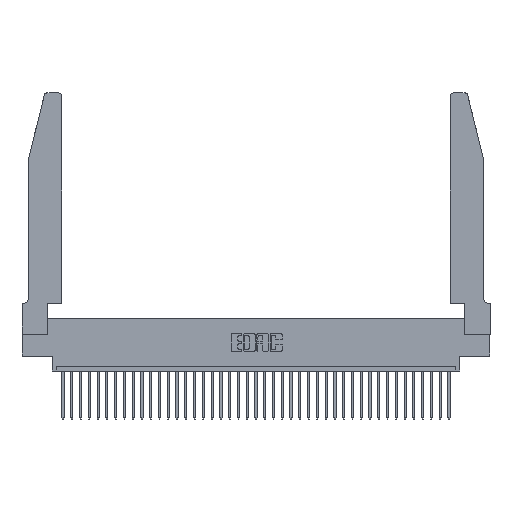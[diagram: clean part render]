
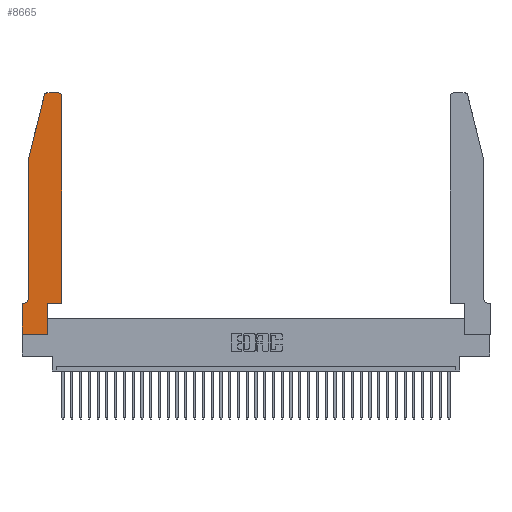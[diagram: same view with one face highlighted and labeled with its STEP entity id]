
A CAD part, top view. The second image highlights one B-rep face of the part: STEP entity #8665.
In plain terms, the highlighted planar face has unit normal (0, 0, 1).
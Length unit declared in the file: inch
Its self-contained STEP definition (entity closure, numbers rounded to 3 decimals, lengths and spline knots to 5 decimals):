
#270 = VECTOR ( 'NONE', #23869, 39.37008 ) ;
#405 = EDGE_LOOP ( 'NONE', ( #17912, #5666, #31619, #15824, #33935, #34351, #32265, #9111, #30380, #34978, #33684, #30118 ) ) ;
#800 = DIRECTION ( 'NONE',  ( -1., 0., 0. ) ) ;
#1045 = FACE_OUTER_BOUND ( 'NONE', #405, .T. ) ;
#1576 = DIRECTION ( 'NONE',  ( 0., 0., 1. ) ) ;
#2291 = DIRECTION ( 'NONE',  ( 1., 0., 0. ) ) ;
#2336 = CARTESIAN_POINT ( 'NONE',  ( 0.0755, 2., 0.37 ) ) ;
#2370 = VERTEX_POINT ( 'NONE', #35701 ) ;
#3829 = EDGE_CURVE ( 'NONE', #26763, #27027, #23783, .T. ) ;
#4012 = DIRECTION ( 'NONE',  ( -1., 0., 0. ) ) ;
#5098 = DIRECTION ( 'NONE',  ( 1., 0., 0. ) ) ;
#5636 = AXIS2_PLACEMENT_3D ( 'NONE', #30112, #15442, #800 ) ;
#5666 = ORIENTED_EDGE ( 'NONE', *, *, #27559, .T. ) ;
#6592 = DIRECTION ( 'NONE',  ( 1., 0., 0. ) ) ;
#6665 = VECTOR ( 'NONE', #4012, 39.37008 ) ;
#6787 = VERTEX_POINT ( 'NONE', #27611 ) ;
#7385 = EDGE_CURVE ( 'NONE', #20689, #2370, #35392, .T. ) ;
#7704 = CARTESIAN_POINT ( 'NONE',  ( 0., 0.35, 0.37 ) ) ;
#7890 = DIRECTION ( 'NONE',  ( 1., 0., 0. ) ) ;
#8224 = LINE ( 'NONE', #18073, #270 ) ;
#8253 = DIRECTION ( 'NONE',  ( 0., 0., 1. ) ) ;
#8665 = ADVANCED_FACE ( 'NONE', ( #1045 ), #26020, .T. ) ;
#9111 = ORIENTED_EDGE ( 'NONE', *, *, #23166, .T. ) ;
#9281 = AXIS2_PLACEMENT_3D ( 'NONE', #11340, #14452, #2291 ) ;
#10300 = CIRCLE ( 'NONE', #5636, 0.07 ) ;
#10449 = VECTOR ( 'NONE', #13274, 39.37008 ) ;
#10702 = CARTESIAN_POINT ( 'NONE',  ( 0.0755, 0.42, 0.37 ) ) ;
#11275 = LINE ( 'NONE', #30943, #25548 ) ;
#11340 = CARTESIAN_POINT ( 'NONE',  ( 0., 0.35, 0.37 ) ) ;
#12788 = EDGE_CURVE ( 'NONE', #31957, #29450, #18213, .T. ) ;
#12957 = VERTEX_POINT ( 'NONE', #33320 ) ;
#13005 = CARTESIAN_POINT ( 'NONE',  ( 0.0755, 2., 0.37 ) ) ;
#13246 = EDGE_CURVE ( 'NONE', #27027, #16882, #38214, .T. ) ;
#13274 = DIRECTION ( 'NONE',  ( 0., -1., 0. ) ) ;
#13630 = DIRECTION ( 'NONE',  ( 0., 1., 0. ) ) ;
#13871 = LINE ( 'NONE', #2336, #31889 ) ;
#14452 = DIRECTION ( 'NONE',  ( 0., 0., 1. ) ) ;
#14983 = VERTEX_POINT ( 'NONE', #33524 ) ;
#15442 = DIRECTION ( 'NONE',  ( 0., 0., -1. ) ) ;
#15448 = CARTESIAN_POINT ( 'NONE',  ( 0.4505, 0.35, 0.37 ) ) ;
#15824 = ORIENTED_EDGE ( 'NONE', *, *, #12788, .T. ) ;
#16882 = VERTEX_POINT ( 'NONE', #15448 ) ;
#17096 = CARTESIAN_POINT ( 'NONE',  ( 0.2865, 0.35, 0.37 ) ) ;
#17912 = ORIENTED_EDGE ( 'NONE', *, *, #7385, .T. ) ;
#18073 = CARTESIAN_POINT ( 'NONE',  ( 0., 0., 0.37 ) ) ;
#18213 = LINE ( 'NONE', #13005, #10449 ) ;
#18218 = CIRCLE ( 'NONE', #29675, 0.03 ) ;
#19226 = CARTESIAN_POINT ( 'NONE',  ( 0.284, 2.72, 0.37 ) ) ;
#19846 = EDGE_CURVE ( 'NONE', #14983, #31957, #13871, .T. ) ;
#20493 = LINE ( 'NONE', #32078, #36821 ) ;
#20689 = VERTEX_POINT ( 'NONE', #32866 ) ;
#20755 = CIRCLE ( 'NONE', #21400, 0.03 ) ;
#21264 = CARTESIAN_POINT ( 'NONE',  ( 0.2865, 0., 0.37 ) ) ;
#21400 = AXIS2_PLACEMENT_3D ( 'NONE', #31741, #8253, #31993 ) ;
#23166 = EDGE_CURVE ( 'NONE', #12957, #26763, #20493, .T. ) ;
#23307 = VECTOR ( 'NONE', #13630, 39.37008 ) ;
#23781 = CARTESIAN_POINT ( 'NONE',  ( 0.2865, 0.35, 0.37 ) ) ;
#23783 = LINE ( 'NONE', #23781, #25234 ) ;
#23869 = DIRECTION ( 'NONE',  ( 0., -1., 0. ) ) ;
#24090 = EDGE_CURVE ( 'NONE', #29450, #6787, #10300, .T. ) ;
#24339 = CARTESIAN_POINT ( 'NONE',  ( 0.2605, 2.75, 0.37 ) ) ;
#24611 = EDGE_CURVE ( 'NONE', #25055, #20689, #20755, .T. ) ;
#24629 = CARTESIAN_POINT ( 'NONE',  ( 0.4505, 0.35, 0.37 ) ) ;
#25055 = VERTEX_POINT ( 'NONE', #35787 ) ;
#25234 = VECTOR ( 'NONE', #31701, 39.37008 ) ;
#25548 = VECTOR ( 'NONE', #30543, 39.37008 ) ;
#26020 = PLANE ( 'NONE',  #9281 ) ;
#26583 = EDGE_CURVE ( 'NONE', #29968, #12957, #8224, .T. ) ;
#26763 = VERTEX_POINT ( 'NONE', #21264 ) ;
#27027 = VERTEX_POINT ( 'NONE', #17096 ) ;
#27559 = EDGE_CURVE ( 'NONE', #2370, #14983, #18218, .T. ) ;
#27611 = CARTESIAN_POINT ( 'NONE',  ( 0.0055, 0.35, 0.37 ) ) ;
#28454 = LINE ( 'NONE', #37430, #23307 ) ;
#29450 = VERTEX_POINT ( 'NONE', #10702 ) ;
#29675 = AXIS2_PLACEMENT_3D ( 'NONE', #19226, #1576, #7890 ) ;
#29968 = VERTEX_POINT ( 'NONE', #7704 ) ;
#30112 = CARTESIAN_POINT ( 'NONE',  ( 0.0055, 0.42, 0.37 ) ) ;
#30118 = ORIENTED_EDGE ( 'NONE', *, *, #24611, .T. ) ;
#30256 = VECTOR ( 'NONE', #6592, 39.37008 ) ;
#30380 = ORIENTED_EDGE ( 'NONE', *, *, #3829, .T. ) ;
#30543 = DIRECTION ( 'NONE',  ( -1., 0., 0. ) ) ;
#30943 = CARTESIAN_POINT ( 'NONE',  ( 0.0755, 0.35, 0.37 ) ) ;
#31619 = ORIENTED_EDGE ( 'NONE', *, *, #19846, .T. ) ;
#31701 = DIRECTION ( 'NONE',  ( 0., 1., 0. ) ) ;
#31741 = CARTESIAN_POINT ( 'NONE',  ( 0.4205, 2.72, 0.37 ) ) ;
#31889 = VECTOR ( 'NONE', #35921, 39.37008 ) ;
#31957 = VERTEX_POINT ( 'NONE', #33663 ) ;
#31993 = DIRECTION ( 'NONE',  ( 1., 0., 0. ) ) ;
#32078 = CARTESIAN_POINT ( 'NONE',  ( 0., 0., 0.37 ) ) ;
#32265 = ORIENTED_EDGE ( 'NONE', *, *, #26583, .T. ) ;
#32550 = EDGE_CURVE ( 'NONE', #16882, #25055, #28454, .T. ) ;
#32866 = CARTESIAN_POINT ( 'NONE',  ( 0.4205, 2.75, 0.37 ) ) ;
#33320 = CARTESIAN_POINT ( 'NONE',  ( 0., 0., 0.37 ) ) ;
#33506 = EDGE_CURVE ( 'NONE', #6787, #29968, #11275, .T. ) ;
#33524 = CARTESIAN_POINT ( 'NONE',  ( 0.25487, 2.72718, 0.37 ) ) ;
#33663 = CARTESIAN_POINT ( 'NONE',  ( 0.0755, 2., 0.37 ) ) ;
#33684 = ORIENTED_EDGE ( 'NONE', *, *, #32550, .T. ) ;
#33935 = ORIENTED_EDGE ( 'NONE', *, *, #24090, .T. ) ;
#34351 = ORIENTED_EDGE ( 'NONE', *, *, #33506, .T. ) ;
#34978 = ORIENTED_EDGE ( 'NONE', *, *, #13246, .T. ) ;
#35392 = LINE ( 'NONE', #24339, #6665 ) ;
#35701 = CARTESIAN_POINT ( 'NONE',  ( 0.284, 2.75, 0.37 ) ) ;
#35787 = CARTESIAN_POINT ( 'NONE',  ( 0.4505, 2.72, 0.37 ) ) ;
#35921 = DIRECTION ( 'NONE',  ( -0.239, -0.971, 0. ) ) ;
#36821 = VECTOR ( 'NONE', #5098, 39.37008 ) ;
#37430 = CARTESIAN_POINT ( 'NONE',  ( 0.4505, 0.35, 0.37 ) ) ;
#38214 = LINE ( 'NONE', #24629, #30256 ) ;
